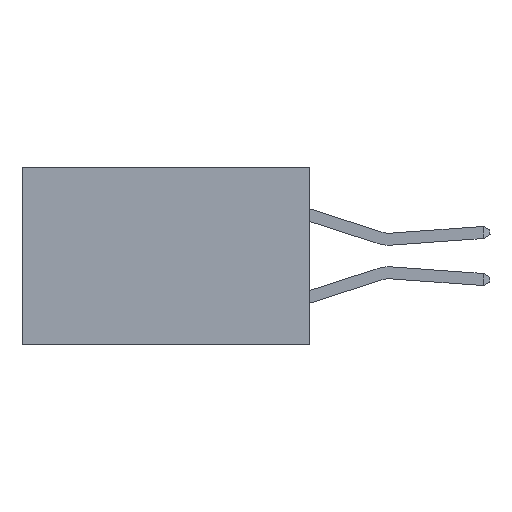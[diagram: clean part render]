
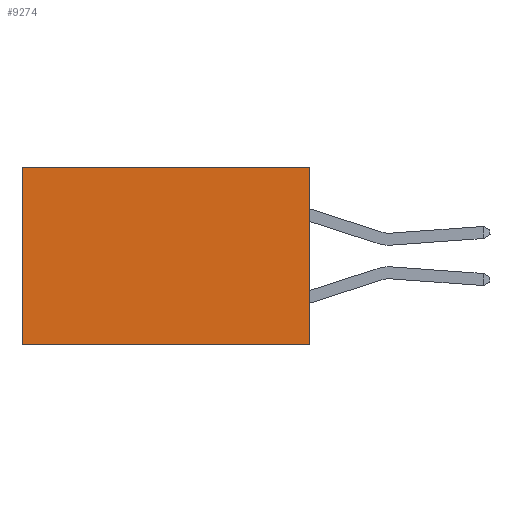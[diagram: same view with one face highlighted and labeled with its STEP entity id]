
A CAD part, left-side view. The second image highlights one B-rep face of the part: STEP entity #9274.
In plain terms, the highlighted planar face has unit normal (-1, 0, 0).
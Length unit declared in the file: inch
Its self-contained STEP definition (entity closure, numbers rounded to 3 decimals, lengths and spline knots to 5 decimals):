
#379 = VERTEX_POINT ( 'NONE', #7023 ) ;
#516 = LINE ( 'NONE', #16936, #8706 ) ;
#541 = CARTESIAN_POINT ( 'NONE',  ( 0.2615, 0., -0.37 ) ) ;
#613 = EDGE_LOOP ( 'NONE', ( #5754, #4377, #17875, #10913 ) ) ;
#991 = EDGE_CURVE ( 'NONE', #379, #18673, #17108, .T. ) ;
#2818 = DIRECTION ( 'NONE',  ( 0., 0., -1. ) ) ;
#3229 = EDGE_CURVE ( 'NONE', #18673, #5768, #8980, .T. ) ;
#3650 = EDGE_CURVE ( 'NONE', #379, #5003, #12594, .T. ) ;
#4240 = CARTESIAN_POINT ( 'NONE',  ( 0.2615, 0.6, -0.37 ) ) ;
#4377 = ORIENTED_EDGE ( 'NONE', *, *, #3229, .F. ) ;
#5003 = VERTEX_POINT ( 'NONE', #8216 ) ;
#5435 = CARTESIAN_POINT ( 'NONE',  ( 0.2615, 0., -0.37 ) ) ;
#5754 = ORIENTED_EDGE ( 'NONE', *, *, #7258, .T. ) ;
#5768 = VERTEX_POINT ( 'NONE', #4240 ) ;
#6387 = AXIS2_PLACEMENT_3D ( 'NONE', #5435, #15533, #8521 ) ;
#7023 = CARTESIAN_POINT ( 'NONE',  ( 0.2615, 0., 0. ) ) ;
#7258 = EDGE_CURVE ( 'NONE', #5003, #5768, #516, .T. ) ;
#8216 = CARTESIAN_POINT ( 'NONE',  ( 0.2615, 0.6, 0. ) ) ;
#8521 = DIRECTION ( 'NONE',  ( 0., 0., -1. ) ) ;
#8522 = VECTOR ( 'NONE', #13959, 39.37008 ) ;
#8706 = VECTOR ( 'NONE', #10251, 39.37008 ) ;
#8980 = LINE ( 'NONE', #541, #8522 ) ;
#9274 = ADVANCED_FACE ( 'NONE', ( #18747 ), #10569, .F. ) ;
#10251 = DIRECTION ( 'NONE',  ( 0., 0., -1. ) ) ;
#10569 = PLANE ( 'NONE',  #6387 ) ;
#10652 = DIRECTION ( 'NONE',  ( 0., 1., 0. ) ) ;
#10913 = ORIENTED_EDGE ( 'NONE', *, *, #3650, .T. ) ;
#11052 = VECTOR ( 'NONE', #2818, 39.37008 ) ;
#12370 = VECTOR ( 'NONE', #10652, 39.37008 ) ;
#12466 = CARTESIAN_POINT ( 'NONE',  ( 0.2615, 0., -0.37 ) ) ;
#12594 = LINE ( 'NONE', #14115, #12370 ) ;
#13651 = CARTESIAN_POINT ( 'NONE',  ( 0.2615, 0., -0.37 ) ) ;
#13959 = DIRECTION ( 'NONE',  ( 0., 1., 0. ) ) ;
#14115 = CARTESIAN_POINT ( 'NONE',  ( 0.2615, 0., 0. ) ) ;
#15533 = DIRECTION ( 'NONE',  ( 1., 0., 0. ) ) ;
#16936 = CARTESIAN_POINT ( 'NONE',  ( 0.2615, 0.6, -0.37 ) ) ;
#17108 = LINE ( 'NONE', #12466, #11052 ) ;
#17875 = ORIENTED_EDGE ( 'NONE', *, *, #991, .F. ) ;
#18673 = VERTEX_POINT ( 'NONE', #13651 ) ;
#18747 = FACE_OUTER_BOUND ( 'NONE', #613, .T. ) ;
